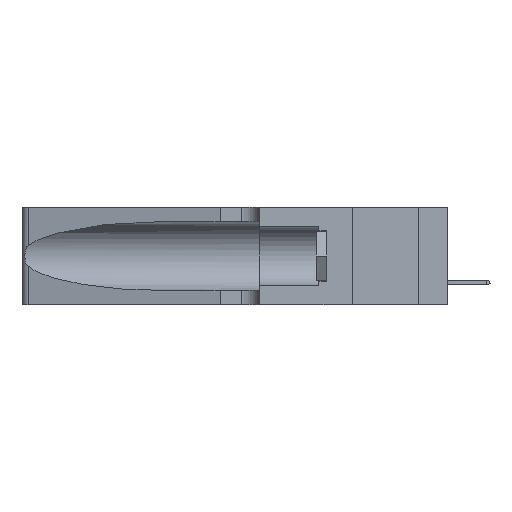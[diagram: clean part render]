
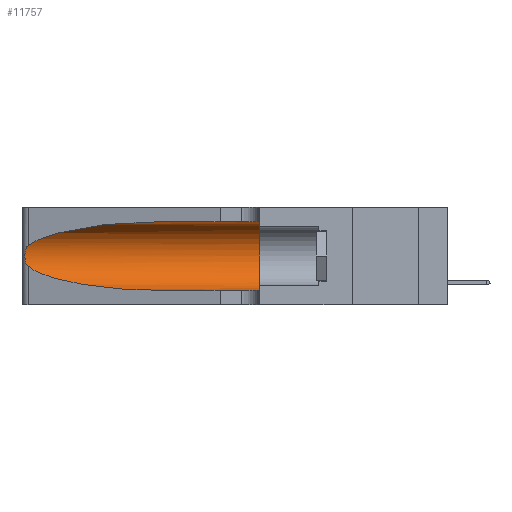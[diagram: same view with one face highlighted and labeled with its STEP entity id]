
A CAD part, left-side view. The second image highlights one B-rep face of the part: STEP entity #11757.
In plain terms, the highlighted cylindrical face has radius 3.308 mm (diameter 6.617 mm), a partial arc.
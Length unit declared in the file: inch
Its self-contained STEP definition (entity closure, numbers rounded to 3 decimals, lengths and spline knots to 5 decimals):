
#743 = DIRECTION ( 'NONE',  ( 0., 0., 1. ) ) ;
#1782 = CARTESIAN_POINT ( 'NONE',  ( 0.18966, 0.96281, 0.31525 ) ) ;
#2745 = CARTESIAN_POINT ( 'NONE',  ( 0.26075, 1.23896, 0.178 ) ) ;
#3108 = LINE ( 'NONE', #13909, #9354 ) ;
#3189 = CARTESIAN_POINT ( 'NONE',  ( 0.1305, 0.35, 0.05475 ) ) ;
#3411 = CARTESIAN_POINT ( 'NONE',  ( 0.18966, 0.96281, 0.05475 ) ) ;
#3512 = AXIS2_PLACEMENT_3D ( 'NONE', #10619, #15879, #743 ) ;
#4033 = CARTESIAN_POINT ( 'NONE',  ( 0.1305, 1.61858, 0.185 ) ) ;
#4087 = VERTEX_POINT ( 'NONE', #16130 ) ;
#4184 = DIRECTION ( 'NONE',  ( 0., -1., 0. ) ) ;
#4280 = CARTESIAN_POINT ( 'NONE',  ( 0.25487, 1.22718, 0.22369 ) ) ;
#4418 = CARTESIAN_POINT ( 'NONE',  ( 0.25856, 1.23593, 0.16098 ) ) ;
#4922 = CARTESIAN_POINT ( 'NONE',  ( 0.2373, 1.15595, 0.28018 ) ) ;
#5258 = CARTESIAN_POINT ( 'NONE',  ( 0.25487, 1.22718, 0.14631 ) ) ;
#5708 = VERTEX_POINT ( 'NONE', #7128 ) ;
#5839 = EDGE_CURVE ( 'NONE', #4087, #15226, #12840, .T. ) ;
#6026 = CARTESIAN_POINT ( 'NONE',  ( 0.25854, 1.2359, 0.20912 ) ) ;
#6132 = ORIENTED_EDGE ( 'NONE', *, *, #5839, .T. ) ;
#6355 = CARTESIAN_POINT ( 'NONE',  ( 0.1305, 1.61858, 0.05475 ) ) ;
#7128 = CARTESIAN_POINT ( 'NONE',  ( 0.1305, 0.72297, 0.05475 ) ) ;
#7245 = EDGE_CURVE ( 'NONE', #4087, #13520, #3108, .T. ) ;
#7424 = ORIENTED_EDGE ( 'NONE', *, *, #20034, .T. ) ;
#8466 = CARTESIAN_POINT ( 'NONE',  ( 0.1305, 0.72297, 0.31525 ) ) ;
#8808 = VERTEX_POINT ( 'NONE', #3189 ) ;
#9354 = VECTOR ( 'NONE', #20639, 39.37008 ) ;
#9572 = CARTESIAN_POINT ( 'NONE',  ( 0.25789, 1.23486, 0.15765 ) ) ;
#9656 = CARTESIAN_POINT ( 'NONE',  ( 0.1305, 0.35, 0.31525 ) ) ;
#9724 = ORIENTED_EDGE ( 'NONE', *, *, #7245, .F. ) ;
#9915 = B_SPLINE_CURVE_WITH_KNOTS ( 'NONE', 3,
 ( #4280, #19207, #11093, #20886, #6026, #21041, #11023, #2745, #14362, #4418, #9572, #12818, #10782, #15794 ),
 .UNSPECIFIED., .F., .F.,
 ( 4, 2, 2, 2, 2, 2, 4 ),
 ( 0., 0.00027, 0.00053, 0.00107, 0.0016, 0.00187, 0.00214 ),
 .UNSPECIFIED. ) ;
#10209 = ORIENTED_EDGE ( 'NONE', *, *, #11829, .T. ) ;
#10321 = CARTESIAN_POINT ( 'NONE',  ( 0.1305, 0.72297, 0.05475 ) ) ;
#10487 = CARTESIAN_POINT ( 'NONE',  ( 0.25487, 1.22718, 0.22369 ) ) ;
#10571 =( BOUNDED_CURVE ( )  B_SPLINE_CURVE ( 3, ( #5258, #13361, #3411, #10321 ),
 .UNSPECIFIED., .F., .F. ) 
 B_SPLINE_CURVE_WITH_KNOTS ( ( 4, 4 ),
 ( 3.44316, 4.71239 ),
 .UNSPECIFIED. ) 
 CURVE ( )  GEOMETRIC_REPRESENTATION_ITEM ( )  RATIONAL_B_SPLINE_CURVE ( ( 1., 0.87, 0.87, 1. ) ) 
 REPRESENTATION_ITEM ( '' )  );
#10619 = CARTESIAN_POINT ( 'NONE',  ( 0.1305, 0.35, 0.185 ) ) ;
#10660 = CIRCLE ( 'NONE', #3512, 0.13025 ) ;
#10782 = CARTESIAN_POINT ( 'NONE',  ( 0.25555, 1.22993, 0.14849 ) ) ;
#11023 = CARTESIAN_POINT ( 'NONE',  ( 0.26075, 1.23896, 0.19203 ) ) ;
#11093 = CARTESIAN_POINT ( 'NONE',  ( 0.25639, 1.23184, 0.21858 ) ) ;
#11132 = EDGE_CURVE ( 'NONE', #15226, #19102, #9915, .T. ) ;
#11498 = ORIENTED_EDGE ( 'NONE', *, *, #19521, .F. ) ;
#11738 = CARTESIAN_POINT ( 'NONE',  ( 0.25487, 1.22718, 0.22369 ) ) ;
#11757 = ADVANCED_FACE ( 'NONE', ( #13037 ), #16968, .F. ) ;
#11829 = EDGE_CURVE ( 'NONE', #5708, #8808, #15382, .T. ) ;
#12818 = CARTESIAN_POINT ( 'NONE',  ( 0.25639, 1.23186, 0.15144 ) ) ;
#12840 =( BOUNDED_CURVE ( )  B_SPLINE_CURVE ( 3, ( #8466, #1782, #4922, #11738 ),
 .UNSPECIFIED., .F., .F. ) 
 B_SPLINE_CURVE_WITH_KNOTS ( ( 4, 4 ),
 ( 1.5708, 2.84003 ),
 .UNSPECIFIED. ) 
 CURVE ( )  GEOMETRIC_REPRESENTATION_ITEM ( )  RATIONAL_B_SPLINE_CURVE ( ( 1., 0.87, 0.87, 1. ) ) 
 REPRESENTATION_ITEM ( '' )  );
#13037 = FACE_OUTER_BOUND ( 'NONE', #16204, .T. ) ;
#13361 = CARTESIAN_POINT ( 'NONE',  ( 0.2373, 1.15595, 0.08982 ) ) ;
#13520 = VERTEX_POINT ( 'NONE', #9656 ) ;
#13909 = CARTESIAN_POINT ( 'NONE',  ( 0.1305, 1.61858, 0.31525 ) ) ;
#14362 = CARTESIAN_POINT ( 'NONE',  ( 0.26017, 1.23833, 0.17102 ) ) ;
#14561 = DIRECTION ( 'NONE',  ( 0., 0., -1. ) ) ;
#15226 = VERTEX_POINT ( 'NONE', #10487 ) ;
#15382 = LINE ( 'NONE', #6355, #17488 ) ;
#15794 = CARTESIAN_POINT ( 'NONE',  ( 0.25487, 1.22718, 0.14631 ) ) ;
#15879 = DIRECTION ( 'NONE',  ( 0., 1., 0. ) ) ;
#16092 = DIRECTION ( 'NONE',  ( 0., -1., 0. ) ) ;
#16130 = CARTESIAN_POINT ( 'NONE',  ( 0.1305, 0.72297, 0.31525 ) ) ;
#16204 = EDGE_LOOP ( 'NONE', ( #6132, #19428, #7424, #10209, #11498, #9724 ) ) ;
#16419 = AXIS2_PLACEMENT_3D ( 'NONE', #4033, #4184, #14561 ) ;
#16741 = CARTESIAN_POINT ( 'NONE',  ( 0.25487, 1.22718, 0.14631 ) ) ;
#16968 = CYLINDRICAL_SURFACE ( 'NONE', #16419, 0.13025 ) ;
#17488 = VECTOR ( 'NONE', #16092, 39.37008 ) ;
#19102 = VERTEX_POINT ( 'NONE', #16741 ) ;
#19207 = CARTESIAN_POINT ( 'NONE',  ( 0.25555, 1.22994, 0.2215 ) ) ;
#19428 = ORIENTED_EDGE ( 'NONE', *, *, #11132, .T. ) ;
#19521 = EDGE_CURVE ( 'NONE', #13520, #8808, #10660, .T. ) ;
#20034 = EDGE_CURVE ( 'NONE', #19102, #5708, #10571, .T. ) ;
#20639 = DIRECTION ( 'NONE',  ( 0., -1., 0. ) ) ;
#20886 = CARTESIAN_POINT ( 'NONE',  ( 0.25787, 1.23484, 0.2124 ) ) ;
#21041 = CARTESIAN_POINT ( 'NONE',  ( 0.26018, 1.23835, 0.19895 ) ) ;
